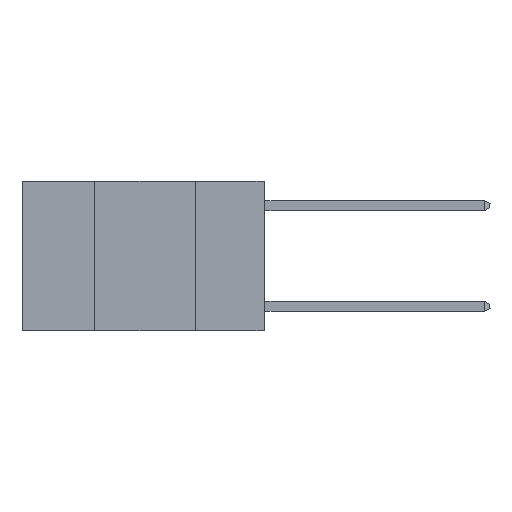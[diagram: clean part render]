
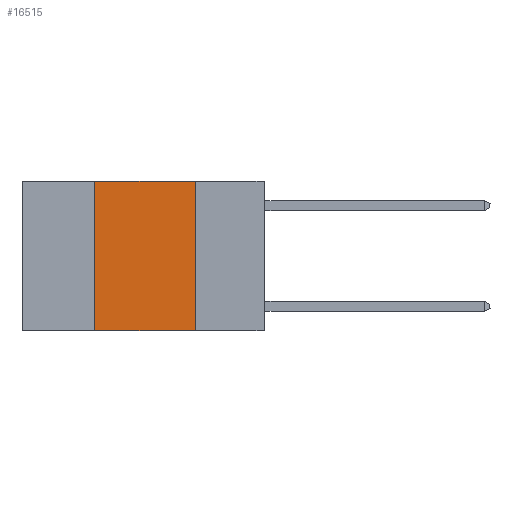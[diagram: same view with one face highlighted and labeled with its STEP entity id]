
A CAD part, left-side view. The second image highlights one B-rep face of the part: STEP entity #16515.
In plain terms, the highlighted planar face has unit normal (-1, 0, 0).
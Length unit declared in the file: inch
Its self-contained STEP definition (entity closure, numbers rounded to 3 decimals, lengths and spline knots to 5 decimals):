
#743 = VERTEX_POINT ( 'NONE', #10776 ) ;
#1448 = VECTOR ( 'NONE', #19103, 39.37008 ) ;
#3120 = FACE_OUTER_BOUND ( 'NONE', #18694, .T. ) ;
#3404 = AXIS2_PLACEMENT_3D ( 'NONE', #15584, #23809, #5234 ) ;
#4300 = ORIENTED_EDGE ( 'NONE', *, *, #6817, .T. ) ;
#5181 = LINE ( 'NONE', #7367, #8797 ) ;
#5234 = DIRECTION ( 'NONE',  ( 0., 0., -1. ) ) ;
#5956 = CARTESIAN_POINT ( 'NONE',  ( 0., 0.17, -0.37 ) ) ;
#6817 = EDGE_CURVE ( 'NONE', #743, #22261, #25182, .T. ) ;
#7185 = VERTEX_POINT ( 'NONE', #10426 ) ;
#7288 = PLANE ( 'NONE',  #3404 ) ;
#7367 = CARTESIAN_POINT ( 'NONE',  ( 0., 0.42, 0. ) ) ;
#8797 = VECTOR ( 'NONE', #19714, 39.37008 ) ;
#8844 = EDGE_CURVE ( 'NONE', #24866, #22261, #13810, .T. ) ;
#10426 = CARTESIAN_POINT ( 'NONE',  ( 0., 0.42, 0. ) ) ;
#10776 = CARTESIAN_POINT ( 'NONE',  ( 0., 0.42, -0.37 ) ) ;
#11454 = VECTOR ( 'NONE', #21493, 39.37008 ) ;
#13810 = LINE ( 'NONE', #26257, #14732 ) ;
#14732 = VECTOR ( 'NONE', #16010, 39.37008 ) ;
#14818 = ORIENTED_EDGE ( 'NONE', *, *, #26668, .F. ) ;
#15179 = CARTESIAN_POINT ( 'NONE',  ( 0., 0.6, -0.37 ) ) ;
#15584 = CARTESIAN_POINT ( 'NONE',  ( 0., 0.6, 0. ) ) ;
#16010 = DIRECTION ( 'NONE',  ( 0., 0., -1. ) ) ;
#16515 = ADVANCED_FACE ( 'NONE', ( #3120 ), #7288, .F. ) ;
#16878 = ORIENTED_EDGE ( 'NONE', *, *, #25620, .F. ) ;
#17054 = LINE ( 'NONE', #19501, #11454 ) ;
#18694 = EDGE_LOOP ( 'NONE', ( #25391, #16878, #14818, #4300 ) ) ;
#19103 = DIRECTION ( 'NONE',  ( 0., -1., 0. ) ) ;
#19501 = CARTESIAN_POINT ( 'NONE',  ( 0., 0.6, 0. ) ) ;
#19714 = DIRECTION ( 'NONE',  ( 0., 0., 1. ) ) ;
#21493 = DIRECTION ( 'NONE',  ( 0., -1., 0. ) ) ;
#22261 = VERTEX_POINT ( 'NONE', #5956 ) ;
#23809 = DIRECTION ( 'NONE',  ( 1., 0., 0. ) ) ;
#24866 = VERTEX_POINT ( 'NONE', #26174 ) ;
#25182 = LINE ( 'NONE', #15179, #1448 ) ;
#25391 = ORIENTED_EDGE ( 'NONE', *, *, #8844, .F. ) ;
#25620 = EDGE_CURVE ( 'NONE', #7185, #24866, #17054, .T. ) ;
#26174 = CARTESIAN_POINT ( 'NONE',  ( 0., 0.17, 0. ) ) ;
#26257 = CARTESIAN_POINT ( 'NONE',  ( 0., 0.17, 0. ) ) ;
#26668 = EDGE_CURVE ( 'NONE', #743, #7185, #5181, .T. ) ;
